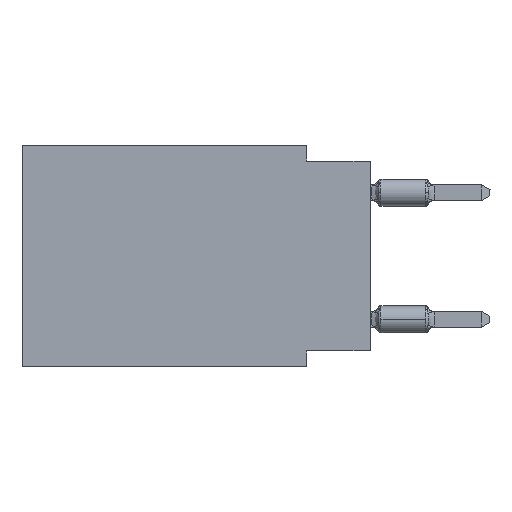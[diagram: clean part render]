
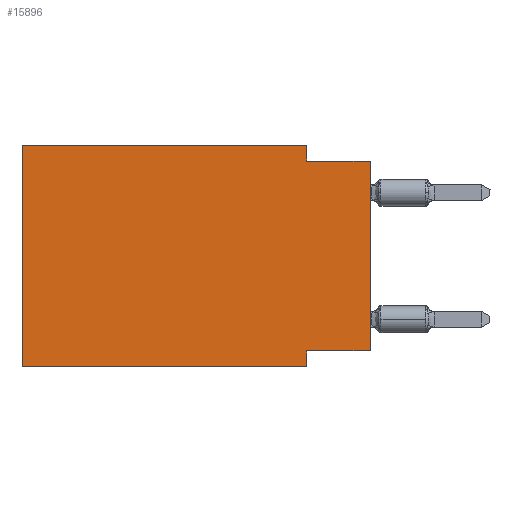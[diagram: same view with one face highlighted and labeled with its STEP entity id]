
A CAD part, left-side view. The second image highlights one B-rep face of the part: STEP entity #15896.
In plain terms, the highlighted planar face has unit normal (-1, 0, 0).
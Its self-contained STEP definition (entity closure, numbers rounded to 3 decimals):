
#352 = CARTESIAN_POINT ( 'NONE',  ( 0., 0., -8.255 ) ) ;
#396 = ORIENTED_EDGE ( 'NONE', *, *, #19111, .T. ) ;
#491 = CARTESIAN_POINT ( 'NONE',  ( 0., 13.97, 0. ) ) ;
#2153 = CARTESIAN_POINT ( 'NONE',  ( 0., 0., -0.635 ) ) ;
#2395 = EDGE_CURVE ( 'NONE', #16189, #3168, #5004, .T. ) ;
#2662 = AXIS2_PLACEMENT_3D ( 'NONE', #5550, #16380, #14515 ) ;
#2862 = DIRECTION ( 'NONE',  ( 0., 0., -1. ) ) ;
#2889 = CARTESIAN_POINT ( 'NONE',  ( 0., 13.97, -8.89 ) ) ;
#3051 = CARTESIAN_POINT ( 'NONE',  ( 0., 0., -0.635 ) ) ;
#3090 = LINE ( 'NONE', #11598, #12246 ) ;
#3168 = VERTEX_POINT ( 'NONE', #3051 ) ;
#3649 = CARTESIAN_POINT ( 'NONE',  ( 0., 13.97, 0. ) ) ;
#4882 = DIRECTION ( 'NONE',  ( 0., 0., 1. ) ) ;
#5004 = LINE ( 'NONE', #8965, #9927 ) ;
#5040 = VECTOR ( 'NONE', #12073, 1000. ) ;
#5453 = VERTEX_POINT ( 'NONE', #8915 ) ;
#5550 = CARTESIAN_POINT ( 'NONE',  ( 0., 13.97, 0. ) ) ;
#5622 = CARTESIAN_POINT ( 'NONE',  ( 0., 2.54, -8.89 ) ) ;
#5866 = VECTOR ( 'NONE', #14562, 1000. ) ;
#6042 = CARTESIAN_POINT ( 'NONE',  ( 0., 13.97, -8.89 ) ) ;
#6094 = VECTOR ( 'NONE', #9125, 1000. ) ;
#6944 = VERTEX_POINT ( 'NONE', #2889 ) ;
#7384 = LINE ( 'NONE', #5622, #15021 ) ;
#7403 = VERTEX_POINT ( 'NONE', #8462 ) ;
#7413 = LINE ( 'NONE', #2153, #14061 ) ;
#7524 = DIRECTION ( 'NONE',  ( 0., -1., 0. ) ) ;
#7725 = VECTOR ( 'NONE', #16652, 1000. ) ;
#8447 = EDGE_CURVE ( 'NONE', #7403, #16128, #3090, .T. ) ;
#8462 = CARTESIAN_POINT ( 'NONE',  ( 0., 2.54, 0. ) ) ;
#8915 = CARTESIAN_POINT ( 'NONE',  ( 0., 2.54, -8.255 ) ) ;
#8965 = CARTESIAN_POINT ( 'NONE',  ( 0., 0., 0. ) ) ;
#9125 = DIRECTION ( 'NONE',  ( 0., 0., 1. ) ) ;
#9226 = ORIENTED_EDGE ( 'NONE', *, *, #10265, .F. ) ;
#9505 = FACE_OUTER_BOUND ( 'NONE', #17128, .T. ) ;
#9927 = VECTOR ( 'NONE', #4882, 1000. ) ;
#10200 = ORIENTED_EDGE ( 'NONE', *, *, #22418, .F. ) ;
#10265 = EDGE_CURVE ( 'NONE', #10946, #7403, #15451, .T. ) ;
#10517 = ORIENTED_EDGE ( 'NONE', *, *, #2395, .T. ) ;
#10937 = VERTEX_POINT ( 'NONE', #10977 ) ;
#10946 = VERTEX_POINT ( 'NONE', #491 ) ;
#10977 = CARTESIAN_POINT ( 'NONE',  ( 0., 2.54, -8.89 ) ) ;
#11598 = CARTESIAN_POINT ( 'NONE',  ( 0., 2.54, 0. ) ) ;
#12073 = DIRECTION ( 'NONE',  ( 0., -1., 0. ) ) ;
#12169 = CARTESIAN_POINT ( 'NONE',  ( 0., 2.54, -0.635 ) ) ;
#12246 = VECTOR ( 'NONE', #2862, 1000. ) ;
#13328 = EDGE_CURVE ( 'NONE', #6944, #10946, #14360, .T. ) ;
#13387 = LINE ( 'NONE', #6042, #7725 ) ;
#13408 = EDGE_CURVE ( 'NONE', #5453, #10937, #7384, .T. ) ;
#13782 = ORIENTED_EDGE ( 'NONE', *, *, #13328, .F. ) ;
#14061 = VECTOR ( 'NONE', #7524, 1000. ) ;
#14360 = LINE ( 'NONE', #3649, #6094 ) ;
#14515 = DIRECTION ( 'NONE',  ( 0., 0., -1. ) ) ;
#14562 = DIRECTION ( 'NONE',  ( 0., 1., 0. ) ) ;
#14743 = PLANE ( 'NONE',  #2662 ) ;
#15021 = VECTOR ( 'NONE', #19850, 1000. ) ;
#15451 = LINE ( 'NONE', #17436, #5040 ) ;
#15896 = ADVANCED_FACE ( 'NONE', ( #9505 ), #14743, .F. ) ;
#16128 = VERTEX_POINT ( 'NONE', #12169 ) ;
#16189 = VERTEX_POINT ( 'NONE', #19169 ) ;
#16380 = DIRECTION ( 'NONE',  ( 1., 0., 0. ) ) ;
#16652 = DIRECTION ( 'NONE',  ( 0., -1., 0. ) ) ;
#17128 = EDGE_LOOP ( 'NONE', ( #10517, #10200, #17725, #9226, #13782, #396, #18251, #18866 ) ) ;
#17436 = CARTESIAN_POINT ( 'NONE',  ( 0., 13.97, 0. ) ) ;
#17725 = ORIENTED_EDGE ( 'NONE', *, *, #8447, .F. ) ;
#18063 = LINE ( 'NONE', #352, #5866 ) ;
#18251 = ORIENTED_EDGE ( 'NONE', *, *, #13408, .F. ) ;
#18866 = ORIENTED_EDGE ( 'NONE', *, *, #21964, .F. ) ;
#19111 = EDGE_CURVE ( 'NONE', #6944, #10937, #13387, .T. ) ;
#19169 = CARTESIAN_POINT ( 'NONE',  ( 0., 0., -8.255 ) ) ;
#19850 = DIRECTION ( 'NONE',  ( 0., 0., -1. ) ) ;
#21964 = EDGE_CURVE ( 'NONE', #16189, #5453, #18063, .T. ) ;
#22418 = EDGE_CURVE ( 'NONE', #16128, #3168, #7413, .T. ) ;
